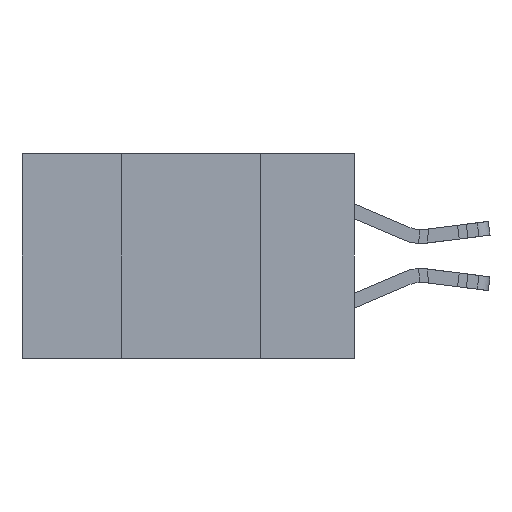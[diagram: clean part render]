
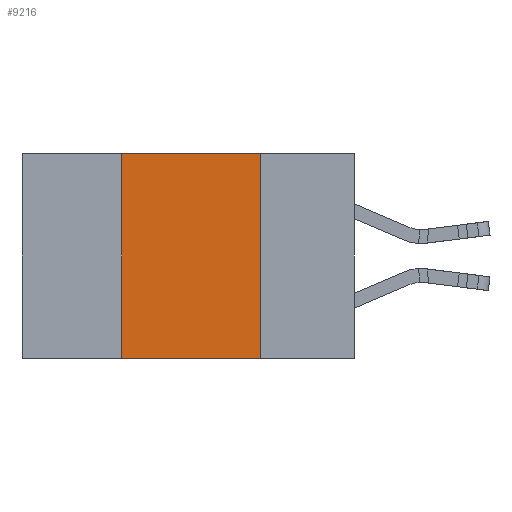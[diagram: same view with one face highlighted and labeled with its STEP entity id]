
A CAD part, left-side view. The second image highlights one B-rep face of the part: STEP entity #9216.
In plain terms, the highlighted planar face has unit normal (-1, 0, 0).
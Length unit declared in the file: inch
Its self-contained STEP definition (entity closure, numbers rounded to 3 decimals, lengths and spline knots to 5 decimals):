
#678 = PLANE ( 'NONE',  #7379 ) ;
#2083 = ORIENTED_EDGE ( 'NONE', *, *, #3370, .T. ) ;
#2270 = LINE ( 'NONE', #25256, #23122 ) ;
#2275 = CARTESIAN_POINT ( 'NONE',  ( 0., 0.42, 0. ) ) ;
#2785 = DIRECTION ( 'NONE',  ( 1., 0., 0. ) ) ;
#2798 = VERTEX_POINT ( 'NONE', #2275 ) ;
#2804 = DIRECTION ( 'NONE',  ( 0., 0., -1. ) ) ;
#3370 = EDGE_CURVE ( 'NONE', #11871, #15458, #2270, .T. ) ;
#3371 = VECTOR ( 'NONE', #2804, 39.37008 ) ;
#4023 = LINE ( 'NONE', #15337, #3371 ) ;
#4082 = DIRECTION ( 'NONE',  ( 0., -1., 0. ) ) ;
#6340 = ORIENTED_EDGE ( 'NONE', *, *, #22031, .F. ) ;
#6411 = FACE_OUTER_BOUND ( 'NONE', #11802, .T. ) ;
#7379 = AXIS2_PLACEMENT_3D ( 'NONE', #15323, #2785, #17398 ) ;
#7815 = LINE ( 'NONE', #8201, #22445 ) ;
#7891 = VECTOR ( 'NONE', #23800, 39.37008 ) ;
#8201 = CARTESIAN_POINT ( 'NONE',  ( 0., 0.6, 0. ) ) ;
#8992 = ORIENTED_EDGE ( 'NONE', *, *, #10930, .F. ) ;
#9216 = ADVANCED_FACE ( 'NONE', ( #6411 ), #678, .F. ) ;
#10930 = EDGE_CURVE ( 'NONE', #22535, #15458, #4023, .T. ) ;
#11087 = CARTESIAN_POINT ( 'NONE',  ( 0., 0.17, 0. ) ) ;
#11802 = EDGE_LOOP ( 'NONE', ( #8992, #24245, #6340, #2083 ) ) ;
#11871 = VERTEX_POINT ( 'NONE', #16022 ) ;
#15323 = CARTESIAN_POINT ( 'NONE',  ( 0., 0.6, 0. ) ) ;
#15337 = CARTESIAN_POINT ( 'NONE',  ( 0., 0.17, -0.37 ) ) ;
#15458 = VERTEX_POINT ( 'NONE', #26035 ) ;
#16022 = CARTESIAN_POINT ( 'NONE',  ( 0., 0.42, -0.37 ) ) ;
#17398 = DIRECTION ( 'NONE',  ( 0., 0., -1. ) ) ;
#17877 = EDGE_CURVE ( 'NONE', #2798, #22535, #7815, .T. ) ;
#19608 = LINE ( 'NONE', #23978, #7891 ) ;
#22031 = EDGE_CURVE ( 'NONE', #11871, #2798, #19608, .T. ) ;
#22445 = VECTOR ( 'NONE', #4082, 39.37008 ) ;
#22535 = VERTEX_POINT ( 'NONE', #11087 ) ;
#23122 = VECTOR ( 'NONE', #24434, 39.37008 ) ;
#23800 = DIRECTION ( 'NONE',  ( 0., 0., 1. ) ) ;
#23978 = CARTESIAN_POINT ( 'NONE',  ( 0., 0.42, -0.37 ) ) ;
#24245 = ORIENTED_EDGE ( 'NONE', *, *, #17877, .F. ) ;
#24434 = DIRECTION ( 'NONE',  ( 0., -1., 0. ) ) ;
#25256 = CARTESIAN_POINT ( 'NONE',  ( 0., 0.6, -0.37 ) ) ;
#26035 = CARTESIAN_POINT ( 'NONE',  ( 0., 0.17, -0.37 ) ) ;
